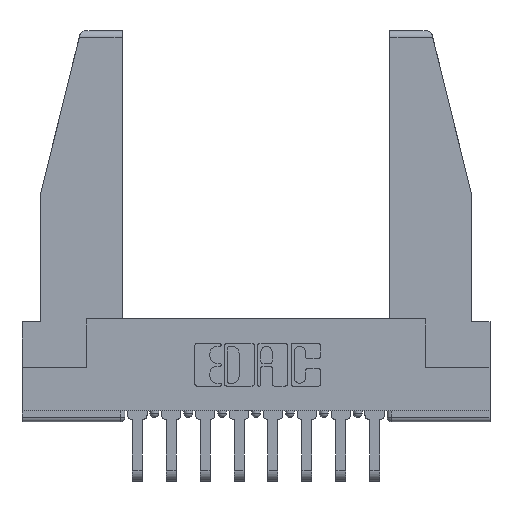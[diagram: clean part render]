
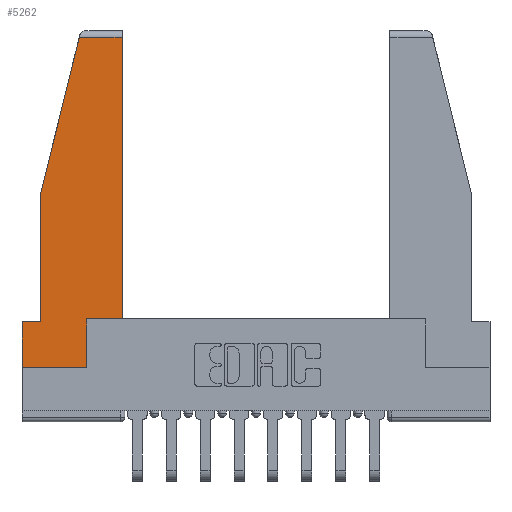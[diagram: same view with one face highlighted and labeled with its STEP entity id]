
A CAD part, top view. The second image highlights one B-rep face of the part: STEP entity #5262.
In plain terms, the highlighted planar face has unit normal (0, 0, 1).
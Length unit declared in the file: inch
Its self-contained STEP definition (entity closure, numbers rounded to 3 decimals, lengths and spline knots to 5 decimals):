
#229 = DIRECTION ( 'NONE',  ( 0., -1., 0. ) ) ;
#307 = DIRECTION ( 'NONE',  ( -1., 0., 0. ) ) ;
#391 = EDGE_CURVE ( 'NONE', #1308, #4255, #3572, .T. ) ;
#394 = CARTESIAN_POINT ( 'NONE',  ( 0., 0., 0. ) ) ;
#495 = CARTESIAN_POINT ( 'NONE',  ( 0.297, 0., 0. ) ) ;
#855 = AXIS2_PLACEMENT_3D ( 'NONE', #12165, #13037, #11060 ) ;
#901 = EDGE_CURVE ( 'NONE', #10010, #4651, #6947, .T. ) ;
#991 = LINE ( 'NONE', #5432, #11396 ) ;
#1056 = VERTEX_POINT ( 'NONE', #13163 ) ;
#1308 = VERTEX_POINT ( 'NONE', #1539 ) ;
#1373 = ORIENTED_EDGE ( 'NONE', *, *, #7757, .T. ) ;
#1539 = CARTESIAN_POINT ( 'NONE',  ( 0.297, 0.223, 0. ) ) ;
#1708 = ORIENTED_EDGE ( 'NONE', *, *, #8064, .T. ) ;
#1934 = FACE_OUTER_BOUND ( 'NONE', #8150, .T. ) ;
#2996 = CARTESIAN_POINT ( 'NONE',  ( 0., 0., 0. ) ) ;
#3201 = EDGE_CURVE ( 'NONE', #5493, #3420, #5007, .T. ) ;
#3420 = VERTEX_POINT ( 'NONE', #6248 ) ;
#3452 = CARTESIAN_POINT ( 'NONE',  ( 0., 1.52, 0. ) ) ;
#3572 = LINE ( 'NONE', #6107, #8378 ) ;
#4141 = VECTOR ( 'NONE', #5385, 39.37008 ) ;
#4255 = VERTEX_POINT ( 'NONE', #5342 ) ;
#4509 = ORIENTED_EDGE ( 'NONE', *, *, #3201, .T. ) ;
#4579 = EDGE_CURVE ( 'NONE', #3420, #8955, #5923, .T. ) ;
#4651 = VERTEX_POINT ( 'NONE', #9584 ) ;
#5007 = LINE ( 'NONE', #6233, #12546 ) ;
#5030 = VECTOR ( 'NONE', #8018, 39.37008 ) ;
#5262 = ADVANCED_FACE ( 'NONE', ( #1934 ), #10097, .T. ) ;
#5342 = CARTESIAN_POINT ( 'NONE',  ( 0.461, 0.223, 0. ) ) ;
#5385 = DIRECTION ( 'NONE',  ( -0.239, -0.971, 0. ) ) ;
#5432 = CARTESIAN_POINT ( 'NONE',  ( 0.297, 0., 0. ) ) ;
#5493 = VERTEX_POINT ( 'NONE', #9159 ) ;
#5897 = CARTESIAN_POINT ( 'NONE',  ( 0.461, 0.223, 0. ) ) ;
#5923 = LINE ( 'NONE', #10644, #8084 ) ;
#6107 = CARTESIAN_POINT ( 'NONE',  ( 0.297, 0.223, 0. ) ) ;
#6233 = CARTESIAN_POINT ( 'NONE',  ( 0., 0.21, 0. ) ) ;
#6248 = CARTESIAN_POINT ( 'NONE',  ( 0., 0.21, 0. ) ) ;
#6262 = ORIENTED_EDGE ( 'NONE', *, *, #391, .T. ) ;
#6464 = ORIENTED_EDGE ( 'NONE', *, *, #7560, .T. ) ;
#6947 = LINE ( 'NONE', #10716, #4141 ) ;
#6949 = EDGE_CURVE ( 'NONE', #4651, #5493, #7519, .T. ) ;
#6956 = LINE ( 'NONE', #3452, #7124 ) ;
#6985 = VERTEX_POINT ( 'NONE', #495 ) ;
#7055 = CARTESIAN_POINT ( 'NONE',  ( 0.2636, 1.52, 0. ) ) ;
#7124 = VECTOR ( 'NONE', #307, 39.37008 ) ;
#7519 = LINE ( 'NONE', #8702, #8336 ) ;
#7560 = EDGE_CURVE ( 'NONE', #8955, #6985, #10927, .T. ) ;
#7757 = EDGE_CURVE ( 'NONE', #6985, #1308, #991, .T. ) ;
#7805 = DIRECTION ( 'NONE',  ( 1., 0., 0. ) ) ;
#8018 = DIRECTION ( 'NONE',  ( 0., 1., 0. ) ) ;
#8064 = EDGE_CURVE ( 'NONE', #1056, #10010, #6956, .T. ) ;
#8084 = VECTOR ( 'NONE', #8618, 39.37008 ) ;
#8150 = EDGE_LOOP ( 'NONE', ( #11464, #1708, #13615, #9104, #4509, #10733, #6464, #1373, #6262 ) ) ;
#8336 = VECTOR ( 'NONE', #229, 39.37008 ) ;
#8378 = VECTOR ( 'NONE', #12379, 39.37008 ) ;
#8489 = DIRECTION ( 'NONE',  ( 0., 1., 0. ) ) ;
#8618 = DIRECTION ( 'NONE',  ( 0., -1., 0. ) ) ;
#8702 = CARTESIAN_POINT ( 'NONE',  ( 0.086, 0.8, 0. ) ) ;
#8955 = VERTEX_POINT ( 'NONE', #2996 ) ;
#9104 = ORIENTED_EDGE ( 'NONE', *, *, #6949, .T. ) ;
#9159 = CARTESIAN_POINT ( 'NONE',  ( 0.086, 0.21, 0. ) ) ;
#9343 = LINE ( 'NONE', #5897, #5030 ) ;
#9447 = VECTOR ( 'NONE', #7805, 39.37008 ) ;
#9584 = CARTESIAN_POINT ( 'NONE',  ( 0.086, 0.8, 0. ) ) ;
#10010 = VERTEX_POINT ( 'NONE', #7055 ) ;
#10097 = PLANE ( 'NONE',  #855 ) ;
#10527 = DIRECTION ( 'NONE',  ( -1., 0., 0. ) ) ;
#10644 = CARTESIAN_POINT ( 'NONE',  ( 0., 0.21, 0. ) ) ;
#10716 = CARTESIAN_POINT ( 'NONE',  ( 0.271, 1.55, 0. ) ) ;
#10733 = ORIENTED_EDGE ( 'NONE', *, *, #4579, .T. ) ;
#10927 = LINE ( 'NONE', #394, #9447 ) ;
#11060 = DIRECTION ( 'NONE',  ( 1., 0., 0. ) ) ;
#11396 = VECTOR ( 'NONE', #8489, 39.37008 ) ;
#11464 = ORIENTED_EDGE ( 'NONE', *, *, #12134, .T. ) ;
#12134 = EDGE_CURVE ( 'NONE', #4255, #1056, #9343, .T. ) ;
#12165 = CARTESIAN_POINT ( 'NONE',  ( 0., 0., 0. ) ) ;
#12379 = DIRECTION ( 'NONE',  ( 1., 0., 0. ) ) ;
#12546 = VECTOR ( 'NONE', #10527, 39.37008 ) ;
#13037 = DIRECTION ( 'NONE',  ( 0., 0., 1. ) ) ;
#13163 = CARTESIAN_POINT ( 'NONE',  ( 0.461, 1.52, 0. ) ) ;
#13615 = ORIENTED_EDGE ( 'NONE', *, *, #901, .T. ) ;
